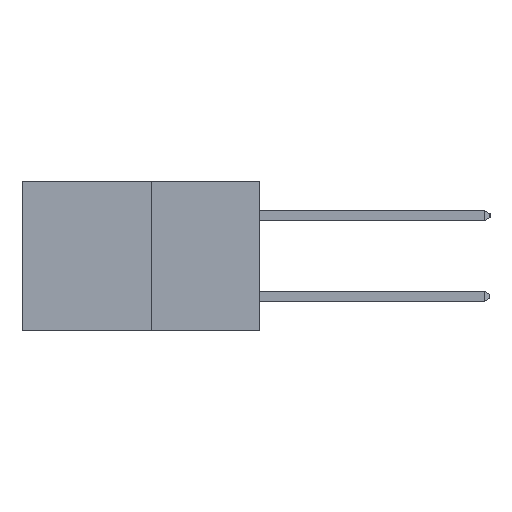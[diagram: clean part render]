
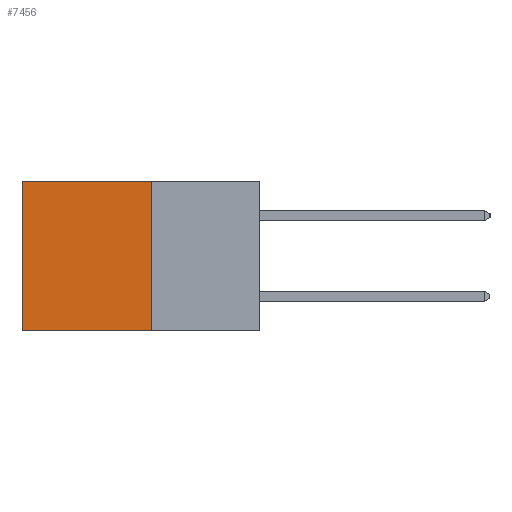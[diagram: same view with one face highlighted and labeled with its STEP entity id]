
A CAD part, left-side view. The second image highlights one B-rep face of the part: STEP entity #7456.
In plain terms, the highlighted planar face has unit normal (-1, 0, 0).
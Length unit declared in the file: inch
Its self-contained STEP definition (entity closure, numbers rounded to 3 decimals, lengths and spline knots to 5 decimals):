
#1016 = EDGE_LOOP ( 'NONE', ( #4485, #6538, #10273, #1672 ) ) ;
#1032 = EDGE_CURVE ( 'NONE', #12490, #11210, #9531, .T. ) ;
#1033 = VECTOR ( 'NONE', #3813, 39.37008 ) ;
#1192 = VERTEX_POINT ( 'NONE', #7943 ) ;
#1221 = LINE ( 'NONE', #4574, #7279 ) ;
#1672 = ORIENTED_EDGE ( 'NONE', *, *, #5910, .T. ) ;
#2606 = CARTESIAN_POINT ( 'NONE',  ( 0.277, 0.27, -0.37 ) ) ;
#2625 = DIRECTION ( 'NONE',  ( 1., 0., 0. ) ) ;
#3458 = DIRECTION ( 'NONE',  ( 0., 0., -1. ) ) ;
#3525 = VECTOR ( 'NONE', #13587, 39.37008 ) ;
#3813 = DIRECTION ( 'NONE',  ( 0., 0., -1. ) ) ;
#3930 = CARTESIAN_POINT ( 'NONE',  ( 0.277, 0.27, -0.37 ) ) ;
#4166 = FACE_OUTER_BOUND ( 'NONE', #1016, .T. ) ;
#4286 = LINE ( 'NONE', #3930, #12916 ) ;
#4426 = CARTESIAN_POINT ( 'NONE',  ( 0.277, 0.59, -0.37 ) ) ;
#4485 = ORIENTED_EDGE ( 'NONE', *, *, #11494, .T. ) ;
#4574 = CARTESIAN_POINT ( 'NONE',  ( 0.277, 0.27, 0. ) ) ;
#4717 = CARTESIAN_POINT ( 'NONE',  ( 0.277, 0.27, -0.37 ) ) ;
#5397 = DIRECTION ( 'NONE',  ( 0., 1., 0. ) ) ;
#5910 = EDGE_CURVE ( 'NONE', #8144, #1192, #1221, .T. ) ;
#6538 = ORIENTED_EDGE ( 'NONE', *, *, #1032, .F. ) ;
#7279 = VECTOR ( 'NONE', #5397, 39.37008 ) ;
#7456 = ADVANCED_FACE ( 'NONE', ( #4166 ), #8624, .F. ) ;
#7943 = CARTESIAN_POINT ( 'NONE',  ( 0.277, 0.59, 0. ) ) ;
#8144 = VERTEX_POINT ( 'NONE', #12994 ) ;
#8562 = CARTESIAN_POINT ( 'NONE',  ( 0.277, 0.59, -0.37 ) ) ;
#8624 = PLANE ( 'NONE',  #11949 ) ;
#9531 = LINE ( 'NONE', #4717, #3525 ) ;
#9655 = EDGE_CURVE ( 'NONE', #8144, #12490, #4286, .T. ) ;
#10273 = ORIENTED_EDGE ( 'NONE', *, *, #9655, .F. ) ;
#11210 = VERTEX_POINT ( 'NONE', #4426 ) ;
#11494 = EDGE_CURVE ( 'NONE', #1192, #11210, #13220, .T. ) ;
#11949 = AXIS2_PLACEMENT_3D ( 'NONE', #2606, #2625, #3458 ) ;
#12490 = VERTEX_POINT ( 'NONE', #14174 ) ;
#12916 = VECTOR ( 'NONE', #14356, 39.37008 ) ;
#12994 = CARTESIAN_POINT ( 'NONE',  ( 0.277, 0.27, 0. ) ) ;
#13220 = LINE ( 'NONE', #8562, #1033 ) ;
#13587 = DIRECTION ( 'NONE',  ( 0., 1., 0. ) ) ;
#14174 = CARTESIAN_POINT ( 'NONE',  ( 0.277, 0.27, -0.37 ) ) ;
#14356 = DIRECTION ( 'NONE',  ( 0., 0., -1. ) ) ;
